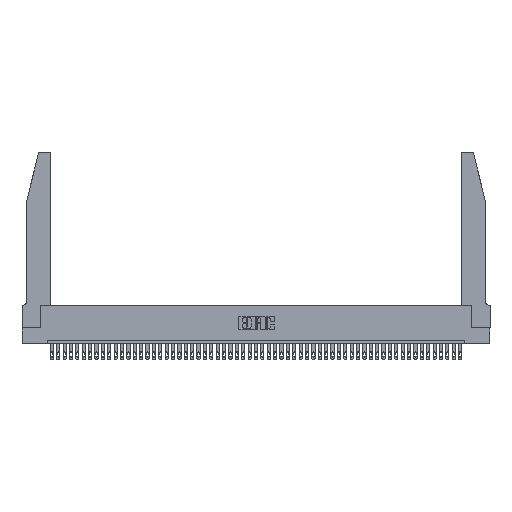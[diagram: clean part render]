
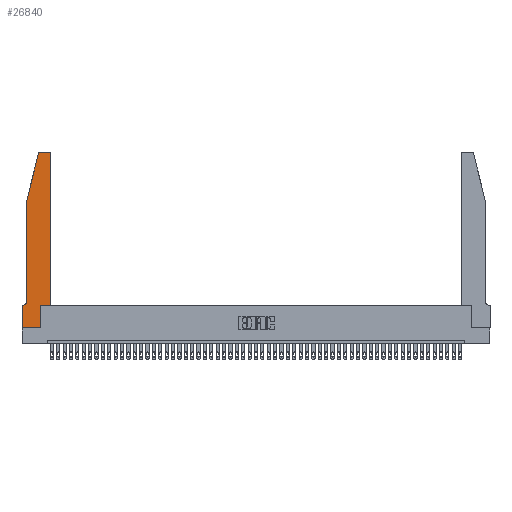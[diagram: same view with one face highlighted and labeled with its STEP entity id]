
A CAD part, top view. The second image highlights one B-rep face of the part: STEP entity #26840.
In plain terms, the highlighted planar face has unit normal (0, 0, 1).
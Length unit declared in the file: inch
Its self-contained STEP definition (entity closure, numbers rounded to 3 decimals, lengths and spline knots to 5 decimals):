
#36 = LINE ( 'NONE', #46215, #20756 ) ;
#3034 = DIRECTION ( 'NONE',  ( 1., 0., 0. ) ) ;
#4671 = VECTOR ( 'NONE', #32554, 39.37008 ) ;
#4681 = CARTESIAN_POINT ( 'NONE',  ( 0.0755, 2., 0.37 ) ) ;
#5664 = CARTESIAN_POINT ( 'NONE',  ( 0.0755, 2., 0.37 ) ) ;
#5779 = ORIENTED_EDGE ( 'NONE', *, *, #15768, .T. ) ;
#5968 = CARTESIAN_POINT ( 'NONE',  ( 0.0755, 2., 0.37 ) ) ;
#7733 = VERTEX_POINT ( 'NONE', #25533 ) ;
#8338 = CARTESIAN_POINT ( 'NONE',  ( 0.4505, 0.35, 0.37 ) ) ;
#8671 = ORIENTED_EDGE ( 'NONE', *, *, #36089, .T. ) ;
#10514 = CARTESIAN_POINT ( 'NONE',  ( 0.2605, 2.75, 0.37 ) ) ;
#10648 = EDGE_CURVE ( 'NONE', #16094, #14388, #36067, .T. ) ;
#11157 = VECTOR ( 'NONE', #20124, 39.37008 ) ;
#11806 = VECTOR ( 'NONE', #29788, 39.37008 ) ;
#11876 = DIRECTION ( 'NONE',  ( 0., 0., 1. ) ) ;
#12364 = ORIENTED_EDGE ( 'NONE', *, *, #34465, .T. ) ;
#12851 = VECTOR ( 'NONE', #18427, 39.37008 ) ;
#13594 = LINE ( 'NONE', #27962, #11157 ) ;
#13646 = DIRECTION ( 'NONE',  ( -1., 0., 0. ) ) ;
#14388 = VERTEX_POINT ( 'NONE', #4681 ) ;
#15378 = ORIENTED_EDGE ( 'NONE', *, *, #35296, .T. ) ;
#15446 = CARTESIAN_POINT ( 'NONE',  ( 0., 0., 0.37 ) ) ;
#15654 = LINE ( 'NONE', #23742, #17455 ) ;
#15716 = VERTEX_POINT ( 'NONE', #49287 ) ;
#15764 = EDGE_CURVE ( 'NONE', #43217, #29020, #15654, .T. ) ;
#15768 = EDGE_CURVE ( 'NONE', #40166, #38006, #38232, .T. ) ;
#16094 = VERTEX_POINT ( 'NONE', #29781 ) ;
#16833 = VECTOR ( 'NONE', #3034, 39.37008 ) ;
#17190 = EDGE_CURVE ( 'NONE', #7733, #32193, #34369, .T. ) ;
#17455 = VECTOR ( 'NONE', #23912, 39.37008 ) ;
#17525 = CARTESIAN_POINT ( 'NONE',  ( 0., 0., 0.37 ) ) ;
#17667 = CARTESIAN_POINT ( 'NONE',  ( 0.4505, 2.72, 0.37 ) ) ;
#17784 = VERTEX_POINT ( 'NONE', #25849 ) ;
#18011 = DIRECTION ( 'NONE',  ( -1., 0., 0. ) ) ;
#18383 = FACE_OUTER_BOUND ( 'NONE', #22260, .T. ) ;
#18427 = DIRECTION ( 'NONE',  ( -0.239, -0.971, 0. ) ) ;
#19490 = CARTESIAN_POINT ( 'NONE',  ( 0.284, 2.75, 0.37 ) ) ;
#19573 = AXIS2_PLACEMENT_3D ( 'NONE', #46164, #30790, #22816 ) ;
#20124 = DIRECTION ( 'NONE',  ( 1., 0., 0. ) ) ;
#20358 = CARTESIAN_POINT ( 'NONE',  ( 0.2865, 0., 0.37 ) ) ;
#20756 = VECTOR ( 'NONE', #26771, 39.37008 ) ;
#21222 = DIRECTION ( 'NONE',  ( 1., 0., 0. ) ) ;
#22028 = VECTOR ( 'NONE', #18011, 39.37008 ) ;
#22260 = EDGE_LOOP ( 'NONE', ( #8671, #44492, #26838, #12364, #43976, #28494, #28910, #15378, #5779, #48010, #24696, #32917 ) ) ;
#22816 = DIRECTION ( 'NONE',  ( 1., 0., 0. ) ) ;
#23742 = CARTESIAN_POINT ( 'NONE',  ( 0.4505, 0.35, 0.37 ) ) ;
#23912 = DIRECTION ( 'NONE',  ( 0., 1., 0. ) ) ;
#24696 = ORIENTED_EDGE ( 'NONE', *, *, #15764, .T. ) ;
#25533 = CARTESIAN_POINT ( 'NONE',  ( 0., 0.35, 0.37 ) ) ;
#25849 = CARTESIAN_POINT ( 'NONE',  ( 0.0055, 0.35, 0.37 ) ) ;
#26771 = DIRECTION ( 'NONE',  ( -1., 0., 0. ) ) ;
#26838 = ORIENTED_EDGE ( 'NONE', *, *, #10648, .T. ) ;
#26840 = ADVANCED_FACE ( 'NONE', ( #18383 ), #39070, .T. ) ;
#27778 = DIRECTION ( 'NONE',  ( 1., 0., 0. ) ) ;
#27962 = CARTESIAN_POINT ( 'NONE',  ( 0., 0., 0.37 ) ) ;
#28494 = ORIENTED_EDGE ( 'NONE', *, *, #28591, .T. ) ;
#28591 = EDGE_CURVE ( 'NONE', #17784, #7733, #36, .T. ) ;
#28910 = ORIENTED_EDGE ( 'NONE', *, *, #17190, .T. ) ;
#29020 = VERTEX_POINT ( 'NONE', #17667 ) ;
#29781 = CARTESIAN_POINT ( 'NONE',  ( 0.25487, 2.72718, 0.37 ) ) ;
#29788 = DIRECTION ( 'NONE',  ( 0., -1., 0. ) ) ;
#30086 = CIRCLE ( 'NONE', #38277, 0.03 ) ;
#30790 = DIRECTION ( 'NONE',  ( 0., 0., 1. ) ) ;
#31927 = CIRCLE ( 'NONE', #19573, 0.03 ) ;
#32193 = VERTEX_POINT ( 'NONE', #15446 ) ;
#32216 = CARTESIAN_POINT ( 'NONE',  ( 0.2865, 0.35, 0.37 ) ) ;
#32554 = DIRECTION ( 'NONE',  ( 0., 1., 0. ) ) ;
#32917 = ORIENTED_EDGE ( 'NONE', *, *, #35004, .T. ) ;
#32923 = DIRECTION ( 'NONE',  ( 0., 0., -1. ) ) ;
#33002 = EDGE_CURVE ( 'NONE', #42463, #16094, #31927, .T. ) ;
#34369 = LINE ( 'NONE', #17525, #11806 ) ;
#34465 = EDGE_CURVE ( 'NONE', #14388, #15716, #48380, .T. ) ;
#35004 = EDGE_CURVE ( 'NONE', #29020, #39673, #30086, .T. ) ;
#35296 = EDGE_CURVE ( 'NONE', #32193, #40166, #13594, .T. ) ;
#35839 = AXIS2_PLACEMENT_3D ( 'NONE', #48618, #32923, #13646 ) ;
#36067 = LINE ( 'NONE', #5664, #12851 ) ;
#36089 = EDGE_CURVE ( 'NONE', #39673, #42463, #40320, .T. ) ;
#36258 = VECTOR ( 'NONE', #37314, 39.37008 ) ;
#36399 = CARTESIAN_POINT ( 'NONE',  ( 0.4205, 2.72, 0.37 ) ) ;
#37314 = DIRECTION ( 'NONE',  ( 0., -1., 0. ) ) ;
#37618 = CARTESIAN_POINT ( 'NONE',  ( 0.2865, 0.35, 0.37 ) ) ;
#37637 = CARTESIAN_POINT ( 'NONE',  ( 0.4205, 2.75, 0.37 ) ) ;
#38006 = VERTEX_POINT ( 'NONE', #37618 ) ;
#38232 = LINE ( 'NONE', #32216, #4671 ) ;
#38277 = AXIS2_PLACEMENT_3D ( 'NONE', #36399, #40317, #21222 ) ;
#39070 = PLANE ( 'NONE',  #45893 ) ;
#39664 = EDGE_CURVE ( 'NONE', #38006, #43217, #41286, .T. ) ;
#39673 = VERTEX_POINT ( 'NONE', #37637 ) ;
#40166 = VERTEX_POINT ( 'NONE', #20358 ) ;
#40317 = DIRECTION ( 'NONE',  ( 0., 0., 1. ) ) ;
#40320 = LINE ( 'NONE', #10514, #22028 ) ;
#41286 = LINE ( 'NONE', #41564, #16833 ) ;
#41564 = CARTESIAN_POINT ( 'NONE',  ( 0.4505, 0.35, 0.37 ) ) ;
#42463 = VERTEX_POINT ( 'NONE', #19490 ) ;
#42718 = CIRCLE ( 'NONE', #35839, 0.07 ) ;
#42799 = CARTESIAN_POINT ( 'NONE',  ( 0., 0.35, 0.37 ) ) ;
#43217 = VERTEX_POINT ( 'NONE', #8338 ) ;
#43976 = ORIENTED_EDGE ( 'NONE', *, *, #49132, .T. ) ;
#44492 = ORIENTED_EDGE ( 'NONE', *, *, #33002, .T. ) ;
#45893 = AXIS2_PLACEMENT_3D ( 'NONE', #42799, #11876, #27778 ) ;
#46164 = CARTESIAN_POINT ( 'NONE',  ( 0.284, 2.72, 0.37 ) ) ;
#46215 = CARTESIAN_POINT ( 'NONE',  ( 0.0755, 0.35, 0.37 ) ) ;
#48010 = ORIENTED_EDGE ( 'NONE', *, *, #39664, .T. ) ;
#48380 = LINE ( 'NONE', #5968, #36258 ) ;
#48618 = CARTESIAN_POINT ( 'NONE',  ( 0.0055, 0.42, 0.37 ) ) ;
#49132 = EDGE_CURVE ( 'NONE', #15716, #17784, #42718, .T. ) ;
#49287 = CARTESIAN_POINT ( 'NONE',  ( 0.0755, 0.42, 0.37 ) ) ;
